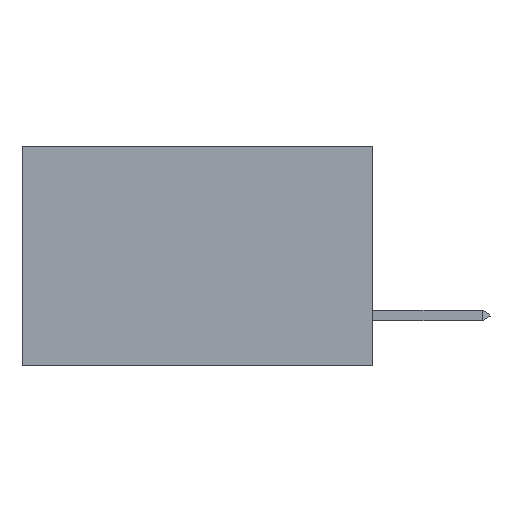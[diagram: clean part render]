
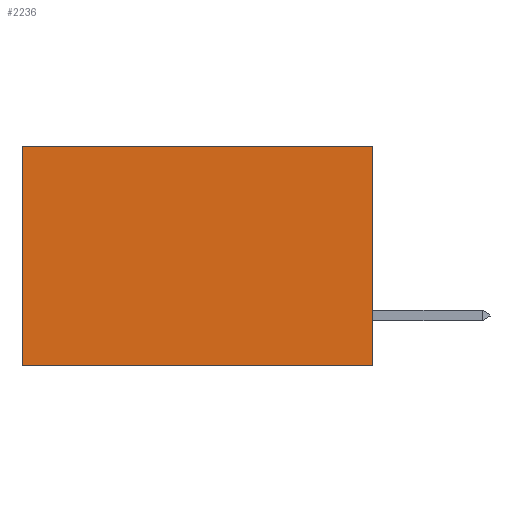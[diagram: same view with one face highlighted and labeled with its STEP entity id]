
A CAD part, left-side view. The second image highlights one B-rep face of the part: STEP entity #2236.
In plain terms, the highlighted planar face has unit normal (-1, 0, 0).
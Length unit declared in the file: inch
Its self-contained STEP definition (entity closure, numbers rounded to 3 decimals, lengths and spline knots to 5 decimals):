
#678 = EDGE_LOOP ( 'NONE', ( #17838, #5827, #10584, #14743 ) ) ;
#771 = FACE_OUTER_BOUND ( 'NONE', #678, .T. ) ;
#850 = LINE ( 'NONE', #7371, #13238 ) ;
#1411 = VECTOR ( 'NONE', #13683, 39.37008 ) ;
#1632 = VECTOR ( 'NONE', #8449, 39.37008 ) ;
#2236 = ADVANCED_FACE ( 'NONE', ( #771 ), #12386, .F. ) ;
#3411 = EDGE_CURVE ( 'NONE', #19076, #15802, #16276, .T. ) ;
#3662 = CARTESIAN_POINT ( 'NONE',  ( 0.277, 0., -0.37 ) ) ;
#4841 = VERTEX_POINT ( 'NONE', #19919 ) ;
#5827 = ORIENTED_EDGE ( 'NONE', *, *, #8469, .F. ) ;
#7227 = AXIS2_PLACEMENT_3D ( 'NONE', #11186, #15767, #9135 ) ;
#7371 = CARTESIAN_POINT ( 'NONE',  ( 0.277, 0.59, -0.37 ) ) ;
#8449 = DIRECTION ( 'NONE',  ( 0., 1., 0. ) ) ;
#8469 = EDGE_CURVE ( 'NONE', #4841, #12518, #11262, .T. ) ;
#9135 = DIRECTION ( 'NONE',  ( 0., 0., -1. ) ) ;
#10033 = LINE ( 'NONE', #12099, #1411 ) ;
#10584 = ORIENTED_EDGE ( 'NONE', *, *, #13106, .F. ) ;
#11186 = CARTESIAN_POINT ( 'NONE',  ( 0.277, 0., -0.37 ) ) ;
#11262 = LINE ( 'NONE', #3662, #1632 ) ;
#12099 = CARTESIAN_POINT ( 'NONE',  ( 0.277, 0., -0.37 ) ) ;
#12171 = DIRECTION ( 'NONE',  ( 0., 0., -1. ) ) ;
#12386 = PLANE ( 'NONE',  #7227 ) ;
#12518 = VERTEX_POINT ( 'NONE', #20223 ) ;
#13106 = EDGE_CURVE ( 'NONE', #19076, #4841, #10033, .T. ) ;
#13146 = EDGE_CURVE ( 'NONE', #15802, #12518, #850, .T. ) ;
#13238 = VECTOR ( 'NONE', #12171, 39.37008 ) ;
#13683 = DIRECTION ( 'NONE',  ( 0., 0., -1. ) ) ;
#14203 = CARTESIAN_POINT ( 'NONE',  ( 0.277, 0., 0. ) ) ;
#14743 = ORIENTED_EDGE ( 'NONE', *, *, #3411, .T. ) ;
#15767 = DIRECTION ( 'NONE',  ( 1., 0., 0. ) ) ;
#15802 = VERTEX_POINT ( 'NONE', #19651 ) ;
#16276 = LINE ( 'NONE', #18595, #18389 ) ;
#16970 = DIRECTION ( 'NONE',  ( 0., 1., 0. ) ) ;
#17838 = ORIENTED_EDGE ( 'NONE', *, *, #13146, .T. ) ;
#18389 = VECTOR ( 'NONE', #16970, 39.37008 ) ;
#18595 = CARTESIAN_POINT ( 'NONE',  ( 0.277, 0., 0. ) ) ;
#19076 = VERTEX_POINT ( 'NONE', #14203 ) ;
#19651 = CARTESIAN_POINT ( 'NONE',  ( 0.277, 0.59, 0. ) ) ;
#19919 = CARTESIAN_POINT ( 'NONE',  ( 0.277, 0., -0.37 ) ) ;
#20223 = CARTESIAN_POINT ( 'NONE',  ( 0.277, 0.59, -0.37 ) ) ;
